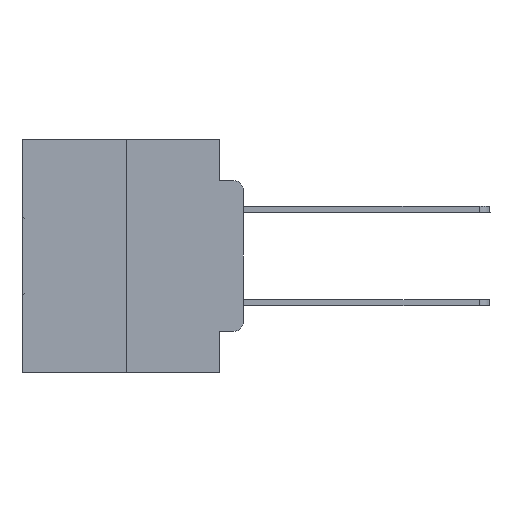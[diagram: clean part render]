
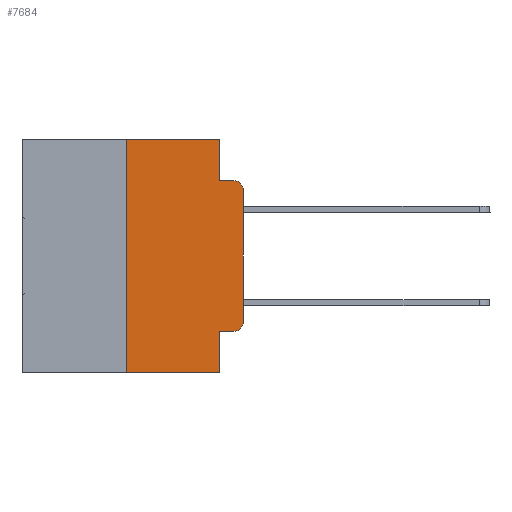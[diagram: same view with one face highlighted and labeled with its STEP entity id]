
A CAD part, left-side view. The second image highlights one B-rep face of the part: STEP entity #7684.
In plain terms, the highlighted planar face has unit normal (-1, 0, 0).
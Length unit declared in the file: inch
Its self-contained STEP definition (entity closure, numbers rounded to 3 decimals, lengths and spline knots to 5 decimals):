
#541 = DIRECTION ( 'NONE',  ( 0., -1., 0. ) ) ;
#1202 = DIRECTION ( 'NONE',  ( 0., -1., 0. ) ) ;
#1585 = EDGE_CURVE ( 'NONE', #30871, #29821, #9431, .T. ) ;
#1851 = CARTESIAN_POINT ( 'NONE',  ( 0., 0.25, 0. ) ) ;
#2565 = ORIENTED_EDGE ( 'NONE', *, *, #7851, .T. ) ;
#2846 = VERTEX_POINT ( 'NONE', #6171 ) ;
#2903 = EDGE_CURVE ( 'NONE', #5942, #3544, #18934, .T. ) ;
#2906 = DIRECTION ( 'NONE',  ( 0., 0., -1. ) ) ;
#3366 = DIRECTION ( 'NONE',  ( 0., 0., 1. ) ) ;
#3413 = ORIENTED_EDGE ( 'NONE', *, *, #1585, .T. ) ;
#3544 = VERTEX_POINT ( 'NONE', #27962 ) ;
#3596 = EDGE_CURVE ( 'NONE', #3544, #26752, #23021, .T. ) ;
#4098 = VECTOR ( 'NONE', #10255, 39.37008 ) ;
#4194 = VECTOR ( 'NONE', #1202, 39.37008 ) ;
#4538 = FACE_OUTER_BOUND ( 'NONE', #29134, .T. ) ;
#5065 = LINE ( 'NONE', #14847, #19219 ) ;
#5246 = CARTESIAN_POINT ( 'NONE',  ( 0., 0.051, -0.0885 ) ) ;
#5411 = CARTESIAN_POINT ( 'NONE',  ( 0., 0.02, -0.3915 ) ) ;
#5942 = VERTEX_POINT ( 'NONE', #31229 ) ;
#5979 = CARTESIAN_POINT ( 'NONE',  ( 0., 0.25, -0.5 ) ) ;
#6100 = CARTESIAN_POINT ( 'NONE',  ( 0., 0., -0.3915 ) ) ;
#6171 = CARTESIAN_POINT ( 'NONE',  ( 0., 0.02, -0.4115 ) ) ;
#6716 = CIRCLE ( 'NONE', #20474, 0.02 ) ;
#7577 = CARTESIAN_POINT ( 'NONE',  ( 0., 0.051, -0.5 ) ) ;
#7684 = ADVANCED_FACE ( 'NONE', ( #4538 ), #32381, .F. ) ;
#7851 = EDGE_CURVE ( 'NONE', #28179, #8632, #31197, .T. ) ;
#8186 = CARTESIAN_POINT ( 'NONE',  ( 0., 0.473, 0. ) ) ;
#8632 = VERTEX_POINT ( 'NONE', #16338 ) ;
#9431 = LINE ( 'NONE', #14758, #22298 ) ;
#10255 = DIRECTION ( 'NONE',  ( 0., 0., -1. ) ) ;
#10959 = VERTEX_POINT ( 'NONE', #20885 ) ;
#11100 = VECTOR ( 'NONE', #26910, 39.37008 ) ;
#11711 = EDGE_CURVE ( 'NONE', #10959, #29821, #19318, .T. ) ;
#11782 = ORIENTED_EDGE ( 'NONE', *, *, #27249, .T. ) ;
#11991 = DIRECTION ( 'NONE',  ( 0., 0., 1. ) ) ;
#12493 = LINE ( 'NONE', #12990, #31234 ) ;
#12609 = DIRECTION ( 'NONE',  ( 0., -1., 0. ) ) ;
#12949 = AXIS2_PLACEMENT_3D ( 'NONE', #5411, #27933, #22498 ) ;
#12990 = CARTESIAN_POINT ( 'NONE',  ( 0., 0.051, -0.4115 ) ) ;
#13034 = CARTESIAN_POINT ( 'NONE',  ( 0., 0.02, -0.1085 ) ) ;
#13249 = CARTESIAN_POINT ( 'NONE',  ( 0., 0.051, 0. ) ) ;
#13599 = EDGE_CURVE ( 'NONE', #10959, #2846, #12493, .T. ) ;
#13977 = CARTESIAN_POINT ( 'NONE',  ( 0., 0.473, 0. ) ) ;
#14036 = CARTESIAN_POINT ( 'NONE',  ( 0., 0.02, -0.0885 ) ) ;
#14758 = CARTESIAN_POINT ( 'NONE',  ( 0., 0.473, -0.5 ) ) ;
#14847 = CARTESIAN_POINT ( 'NONE',  ( 0., 0.051, -0.0885 ) ) ;
#15488 = DIRECTION ( 'NONE',  ( 0., -1., 0. ) ) ;
#16047 = ORIENTED_EDGE ( 'NONE', *, *, #21374, .F. ) ;
#16217 = VECTOR ( 'NONE', #3366, 39.37008 ) ;
#16338 = CARTESIAN_POINT ( 'NONE',  ( 0., 0., -0.1085 ) ) ;
#16840 = ORIENTED_EDGE ( 'NONE', *, *, #13599, .T. ) ;
#17806 = AXIS2_PLACEMENT_3D ( 'NONE', #8186, #31034, #17974 ) ;
#17974 = DIRECTION ( 'NONE',  ( 0., 0., -1. ) ) ;
#18366 = ORIENTED_EDGE ( 'NONE', *, *, #20604, .F. ) ;
#18768 = DIRECTION ( 'NONE',  ( -1., 0., 0. ) ) ;
#18934 = LINE ( 'NONE', #13977, #4194 ) ;
#19219 = VECTOR ( 'NONE', #15488, 39.37008 ) ;
#19318 = LINE ( 'NONE', #19636, #11100 ) ;
#19585 = EDGE_CURVE ( 'NONE', #2846, #28179, #23511, .T. ) ;
#19636 = CARTESIAN_POINT ( 'NONE',  ( 0., 0.051, 0. ) ) ;
#20474 = AXIS2_PLACEMENT_3D ( 'NONE', #13034, #18768, #2906 ) ;
#20604 = EDGE_CURVE ( 'NONE', #30871, #5942, #27847, .T. ) ;
#20885 = CARTESIAN_POINT ( 'NONE',  ( 0., 0.051, -0.4115 ) ) ;
#20939 = CARTESIAN_POINT ( 'NONE',  ( 0., 0., 0. ) ) ;
#21374 = EDGE_CURVE ( 'NONE', #26752, #32094, #5065, .T. ) ;
#22298 = VECTOR ( 'NONE', #12609, 39.37008 ) ;
#22498 = DIRECTION ( 'NONE',  ( 0., 0., -1. ) ) ;
#22709 = ORIENTED_EDGE ( 'NONE', *, *, #19585, .T. ) ;
#22805 = ORIENTED_EDGE ( 'NONE', *, *, #11711, .F. ) ;
#23021 = LINE ( 'NONE', #13249, #4098 ) ;
#23511 = CIRCLE ( 'NONE', #12949, 0.02 ) ;
#26394 = ORIENTED_EDGE ( 'NONE', *, *, #2903, .F. ) ;
#26557 = VECTOR ( 'NONE', #11991, 39.37008 ) ;
#26752 = VERTEX_POINT ( 'NONE', #5246 ) ;
#26910 = DIRECTION ( 'NONE',  ( 0., 0., -1. ) ) ;
#27249 = EDGE_CURVE ( 'NONE', #8632, #32094, #6716, .T. ) ;
#27847 = LINE ( 'NONE', #1851, #26557 ) ;
#27929 = ORIENTED_EDGE ( 'NONE', *, *, #3596, .F. ) ;
#27933 = DIRECTION ( 'NONE',  ( -1., 0., 0. ) ) ;
#27962 = CARTESIAN_POINT ( 'NONE',  ( 0., 0.051, 0. ) ) ;
#28179 = VERTEX_POINT ( 'NONE', #6100 ) ;
#29134 = EDGE_LOOP ( 'NONE', ( #2565, #11782, #16047, #27929, #26394, #18366, #3413, #22805, #16840, #22709 ) ) ;
#29821 = VERTEX_POINT ( 'NONE', #7577 ) ;
#30871 = VERTEX_POINT ( 'NONE', #5979 ) ;
#31034 = DIRECTION ( 'NONE',  ( 1., 0., 0. ) ) ;
#31197 = LINE ( 'NONE', #20939, #16217 ) ;
#31229 = CARTESIAN_POINT ( 'NONE',  ( 0., 0.25, 0. ) ) ;
#31234 = VECTOR ( 'NONE', #541, 39.37008 ) ;
#32094 = VERTEX_POINT ( 'NONE', #14036 ) ;
#32381 = PLANE ( 'NONE',  #17806 ) ;
